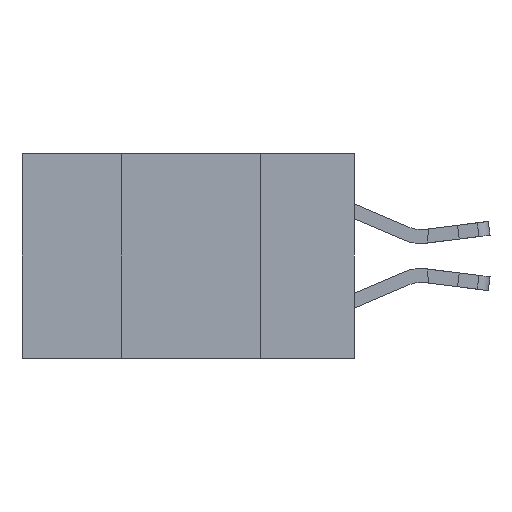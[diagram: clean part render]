
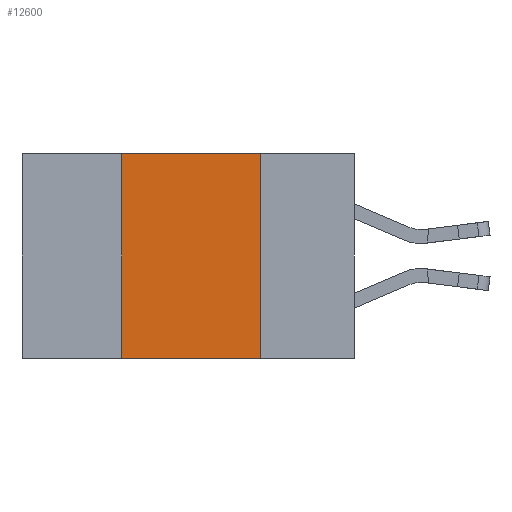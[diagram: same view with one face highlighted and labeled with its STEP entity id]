
A CAD part, left-side view. The second image highlights one B-rep face of the part: STEP entity #12600.
In plain terms, the highlighted planar face has unit normal (-1, 0, 0).
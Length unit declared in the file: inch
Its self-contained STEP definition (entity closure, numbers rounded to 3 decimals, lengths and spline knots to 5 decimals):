
#929 = CARTESIAN_POINT ( 'NONE',  ( 0., 0.42, -0.37 ) ) ;
#993 = EDGE_CURVE ( 'NONE', #12641, #4681, #7288, .T. ) ;
#1057 = CARTESIAN_POINT ( 'NONE',  ( 0., 0.6, 0. ) ) ;
#1146 = EDGE_CURVE ( 'NONE', #2005, #4681, #2989, .T. ) ;
#1739 = EDGE_CURVE ( 'NONE', #5866, #2005, #2991, .T. ) ;
#2005 = VERTEX_POINT ( 'NONE', #9602 ) ;
#2055 = LINE ( 'NONE', #9993, #2225 ) ;
#2225 = VECTOR ( 'NONE', #7840, 39.37008 ) ;
#2409 = ORIENTED_EDGE ( 'NONE', *, *, #1146, .F. ) ;
#2757 = ORIENTED_EDGE ( 'NONE', *, *, #1739, .F. ) ;
#2989 = LINE ( 'NONE', #12896, #8253 ) ;
#2991 = LINE ( 'NONE', #12129, #9093 ) ;
#3529 = DIRECTION ( 'NONE',  ( 0., 0., -1. ) ) ;
#4140 = ORIENTED_EDGE ( 'NONE', *, *, #10292, .F. ) ;
#4681 = VERTEX_POINT ( 'NONE', #10464 ) ;
#5120 = PLANE ( 'NONE',  #10899 ) ;
#5866 = VERTEX_POINT ( 'NONE', #9727 ) ;
#6024 = DIRECTION ( 'NONE',  ( 0., -1., 0. ) ) ;
#7288 = LINE ( 'NONE', #9067, #11249 ) ;
#7840 = DIRECTION ( 'NONE',  ( 0., 0., 1. ) ) ;
#8253 = VECTOR ( 'NONE', #3529, 39.37008 ) ;
#9067 = CARTESIAN_POINT ( 'NONE',  ( 0., 0.6, -0.37 ) ) ;
#9093 = VECTOR ( 'NONE', #12308, 39.37008 ) ;
#9602 = CARTESIAN_POINT ( 'NONE',  ( 0., 0.17, 0. ) ) ;
#9727 = CARTESIAN_POINT ( 'NONE',  ( 0., 0.42, 0. ) ) ;
#9993 = CARTESIAN_POINT ( 'NONE',  ( 0., 0.42, 0. ) ) ;
#10292 = EDGE_CURVE ( 'NONE', #12641, #5866, #2055, .T. ) ;
#10464 = CARTESIAN_POINT ( 'NONE',  ( 0., 0.17, -0.37 ) ) ;
#10509 = DIRECTION ( 'NONE',  ( 1., 0., 0. ) ) ;
#10743 = EDGE_LOOP ( 'NONE', ( #2409, #2757, #4140, #11628 ) ) ;
#10899 = AXIS2_PLACEMENT_3D ( 'NONE', #1057, #10509, #13559 ) ;
#11249 = VECTOR ( 'NONE', #6024, 39.37008 ) ;
#11269 = FACE_OUTER_BOUND ( 'NONE', #10743, .T. ) ;
#11628 = ORIENTED_EDGE ( 'NONE', *, *, #993, .T. ) ;
#12129 = CARTESIAN_POINT ( 'NONE',  ( 0., 0.6, 0. ) ) ;
#12308 = DIRECTION ( 'NONE',  ( 0., -1., 0. ) ) ;
#12600 = ADVANCED_FACE ( 'NONE', ( #11269 ), #5120, .F. ) ;
#12641 = VERTEX_POINT ( 'NONE', #929 ) ;
#12896 = CARTESIAN_POINT ( 'NONE',  ( 0., 0.17, 0. ) ) ;
#13559 = DIRECTION ( 'NONE',  ( 0., 0., -1. ) ) ;
